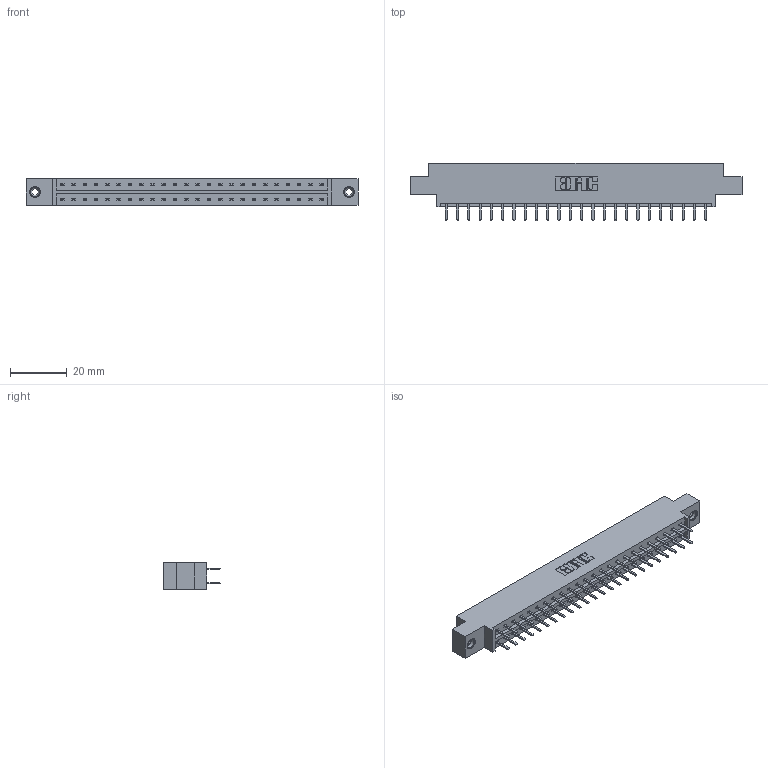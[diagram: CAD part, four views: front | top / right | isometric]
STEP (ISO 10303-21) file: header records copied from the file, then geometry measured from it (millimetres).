
FILE_DESCRIPTION (( 'STEP AP203' ), '1' );
FILE_NAME ('833-048-520-808.STEP', '2020-06-04T15:29:33', ( '' ), ( '' ), 'SwSTEP 2.0', 'SolidWorks 2020', '' );
FILE_SCHEMA (( 'CONFIG_CONTROL_DESIGN' ));
Length unit declared in the file: inch
Products named in the file (4): 833-048-520-808; 345-292-001_345-293-120; 833 Part_Offset - .156 Dia - TI; 345-250-001_345-250-003-102
Assembly tree (51 placements, depth 2):
  833-048-520-808
    833 Part_Offset - .156 Dia - TI
    345-292-001_345-293-120  x48
    345-250-001_345-250-003-102  x2
Bounding box: 116.64 x 20.02 x 9.4 mm (x, y, z)
Volume: 11484.2 mm3; surface area: 13570.5 mm2
Topology: 51 solids, 51 shells, 2866 faces, 8283 edges, 5386 vertices
Faces by surface type: plane 1930, cylinder 920, cone 12, torus 4
Entity records: 19200 total; most frequent: CARTESIAN_POINT 3201, ORIENTED_EDGE 3118, DIRECTION 2785, EDGE_CURVE 1559, VECTOR 1407, LINE 1407, VERTEX_POINT 1032, AXIS2_PLACEMENT_3D 689
